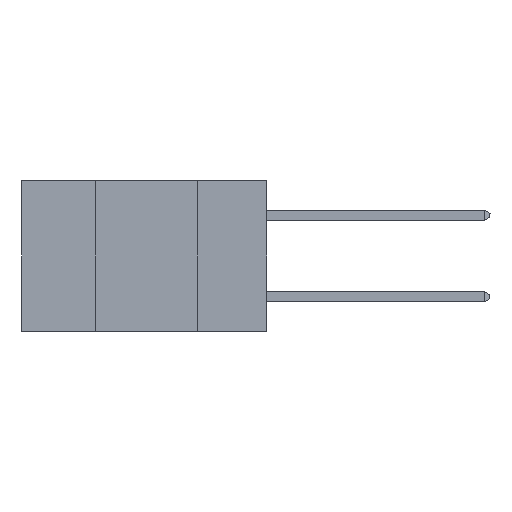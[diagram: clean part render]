
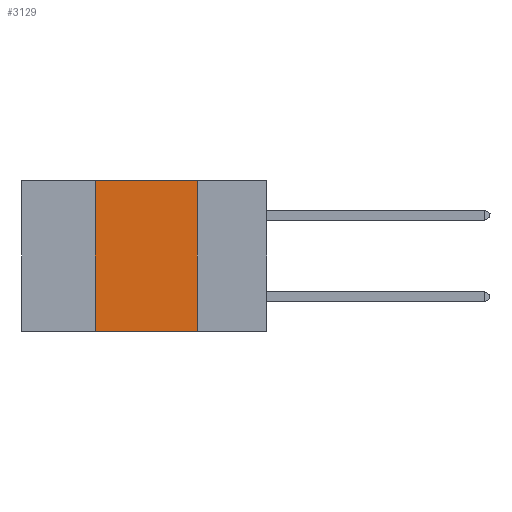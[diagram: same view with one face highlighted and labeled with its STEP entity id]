
A CAD part, left-side view. The second image highlights one B-rep face of the part: STEP entity #3129.
In plain terms, the highlighted planar face has unit normal (-1, 0, 0).
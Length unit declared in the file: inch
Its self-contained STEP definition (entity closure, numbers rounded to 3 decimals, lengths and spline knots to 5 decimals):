
#2894 = VERTEX_POINT ( 'NONE', #21932 ) ;
#2980 = VECTOR ( 'NONE', #7979, 39.37008 ) ;
#3102 = ORIENTED_EDGE ( 'NONE', *, *, #26429, .F. ) ;
#3129 = ADVANCED_FACE ( 'NONE', ( #16412 ), #16355, .F. ) ;
#3168 = CARTESIAN_POINT ( 'NONE',  ( 0., 0.6, 0. ) ) ;
#3415 = VECTOR ( 'NONE', #13581, 39.37008 ) ;
#3679 = VECTOR ( 'NONE', #42702, 39.37008 ) ;
#3964 = LINE ( 'NONE', #13540, #28372 ) ;
#4642 = CARTESIAN_POINT ( 'NONE',  ( 0., 0.42, 0. ) ) ;
#5154 = EDGE_LOOP ( 'NONE', ( #3102, #20294, #38214, #16069 ) ) ;
#6852 = DIRECTION ( 'NONE',  ( 0., -1., 0. ) ) ;
#7979 = DIRECTION ( 'NONE',  ( 0., 0., 1. ) ) ;
#9828 = DIRECTION ( 'NONE',  ( 1., 0., 0. ) ) ;
#10216 = EDGE_CURVE ( 'NONE', #27786, #21280, #21089, .T. ) ;
#10841 = AXIS2_PLACEMENT_3D ( 'NONE', #3168, #9828, #32990 ) ;
#13540 = CARTESIAN_POINT ( 'NONE',  ( 0., 0.6, -0.37 ) ) ;
#13581 = DIRECTION ( 'NONE',  ( 0., -1., 0. ) ) ;
#16069 = ORIENTED_EDGE ( 'NONE', *, *, #21917, .T. ) ;
#16355 = PLANE ( 'NONE',  #10841 ) ;
#16412 = FACE_OUTER_BOUND ( 'NONE', #5154, .T. ) ;
#19587 = CARTESIAN_POINT ( 'NONE',  ( 0., 0.42, 0. ) ) ;
#19808 = CARTESIAN_POINT ( 'NONE',  ( 0., 0.17, 0. ) ) ;
#20294 = ORIENTED_EDGE ( 'NONE', *, *, #10216, .F. ) ;
#21089 = LINE ( 'NONE', #33384, #3415 ) ;
#21280 = VERTEX_POINT ( 'NONE', #31845 ) ;
#21372 = LINE ( 'NONE', #19808, #3679 ) ;
#21917 = EDGE_CURVE ( 'NONE', #25414, #2894, #3964, .T. ) ;
#21932 = CARTESIAN_POINT ( 'NONE',  ( 0., 0.17, -0.37 ) ) ;
#25414 = VERTEX_POINT ( 'NONE', #41048 ) ;
#26429 = EDGE_CURVE ( 'NONE', #21280, #2894, #21372, .T. ) ;
#27786 = VERTEX_POINT ( 'NONE', #19587 ) ;
#28372 = VECTOR ( 'NONE', #6852, 39.37008 ) ;
#29460 = LINE ( 'NONE', #4642, #2980 ) ;
#31845 = CARTESIAN_POINT ( 'NONE',  ( 0., 0.17, 0. ) ) ;
#32990 = DIRECTION ( 'NONE',  ( 0., 0., -1. ) ) ;
#33384 = CARTESIAN_POINT ( 'NONE',  ( 0., 0.6, 0. ) ) ;
#38214 = ORIENTED_EDGE ( 'NONE', *, *, #38454, .F. ) ;
#38454 = EDGE_CURVE ( 'NONE', #25414, #27786, #29460, .T. ) ;
#41048 = CARTESIAN_POINT ( 'NONE',  ( 0., 0.42, -0.37 ) ) ;
#42702 = DIRECTION ( 'NONE',  ( 0., 0., -1. ) ) ;
